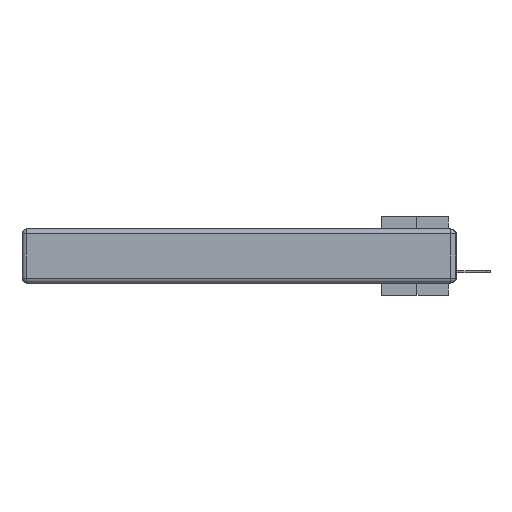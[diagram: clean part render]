
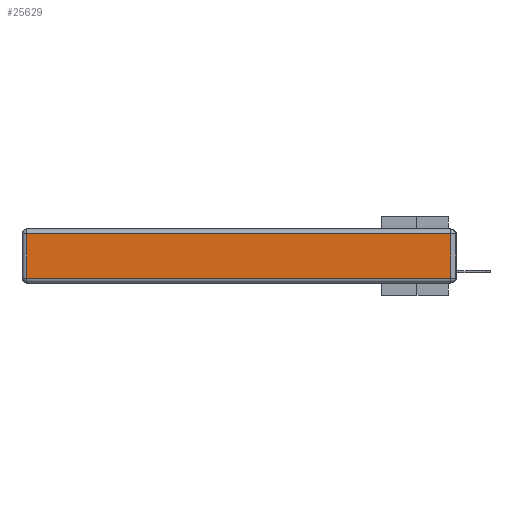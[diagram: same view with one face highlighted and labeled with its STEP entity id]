
A CAD part, left-side view. The second image highlights one B-rep face of the part: STEP entity #25629.
In plain terms, the highlighted planar face has unit normal (-1, 0, 0).
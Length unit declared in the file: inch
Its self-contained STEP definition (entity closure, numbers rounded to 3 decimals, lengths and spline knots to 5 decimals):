
#553 = CARTESIAN_POINT ( 'NONE',  ( 0., 0.03, -0.343 ) ) ;
#977 = CARTESIAN_POINT ( 'NONE',  ( 0., 0.03, -0.313 ) ) ;
#1754 = DIRECTION ( 'NONE',  ( 0., -1., 0. ) ) ;
#2260 = CARTESIAN_POINT ( 'NONE',  ( 0., 0., -0.343 ) ) ;
#3828 = VECTOR ( 'NONE', #1754, 39.37008 ) ;
#4702 = AXIS2_PLACEMENT_3D ( 'NONE', #2260, #16198, #5131 ) ;
#5131 = DIRECTION ( 'NONE',  ( 0., 0., 1. ) ) ;
#7337 = CARTESIAN_POINT ( 'NONE',  ( 0., 2.72, -0.343 ) ) ;
#8582 = LINE ( 'NONE', #15534, #3828 ) ;
#8694 = VERTEX_POINT ( 'NONE', #977 ) ;
#8961 = VECTOR ( 'NONE', #9639, 39.37008 ) ;
#9639 = DIRECTION ( 'NONE',  ( 0., 0., 1. ) ) ;
#10401 = VERTEX_POINT ( 'NONE', #23964 ) ;
#12102 = LINE ( 'NONE', #21331, #16653 ) ;
#13061 = VECTOR ( 'NONE', #16594, 39.37008 ) ;
#14007 = EDGE_LOOP ( 'NONE', ( #21479, #16825, #17251, #26317 ) ) ;
#15534 = CARTESIAN_POINT ( 'NONE',  ( 0., 0., -0.313 ) ) ;
#16198 = DIRECTION ( 'NONE',  ( -1., 0., 0. ) ) ;
#16275 = LINE ( 'NONE', #7337, #13061 ) ;
#16594 = DIRECTION ( 'NONE',  ( 0., 0., -1. ) ) ;
#16653 = VECTOR ( 'NONE', #19038, 39.37008 ) ;
#16825 = ORIENTED_EDGE ( 'NONE', *, *, #23774, .T. ) ;
#17251 = ORIENTED_EDGE ( 'NONE', *, *, #20770, .T. ) ;
#19038 = DIRECTION ( 'NONE',  ( 0., 1., 0. ) ) ;
#19127 = VERTEX_POINT ( 'NONE', #22854 ) ;
#20165 = CARTESIAN_POINT ( 'NONE',  ( 0., 2.72, -0.03 ) ) ;
#20770 = EDGE_CURVE ( 'NONE', #19127, #29132, #12102, .T. ) ;
#21331 = CARTESIAN_POINT ( 'NONE',  ( 0., 2.75, -0.03 ) ) ;
#21479 = ORIENTED_EDGE ( 'NONE', *, *, #27646, .T. ) ;
#22854 = CARTESIAN_POINT ( 'NONE',  ( 0., 0.03, -0.03 ) ) ;
#23318 = PLANE ( 'NONE',  #4702 ) ;
#23774 = EDGE_CURVE ( 'NONE', #8694, #19127, #27823, .T. ) ;
#23964 = CARTESIAN_POINT ( 'NONE',  ( 0., 2.72, -0.313 ) ) ;
#25298 = FACE_OUTER_BOUND ( 'NONE', #14007, .T. ) ;
#25629 = ADVANCED_FACE ( 'NONE', ( #25298 ), #23318, .T. ) ;
#26317 = ORIENTED_EDGE ( 'NONE', *, *, #27839, .T. ) ;
#27646 = EDGE_CURVE ( 'NONE', #10401, #8694, #8582, .T. ) ;
#27823 = LINE ( 'NONE', #553, #8961 ) ;
#27839 = EDGE_CURVE ( 'NONE', #29132, #10401, #16275, .T. ) ;
#29132 = VERTEX_POINT ( 'NONE', #20165 ) ;
